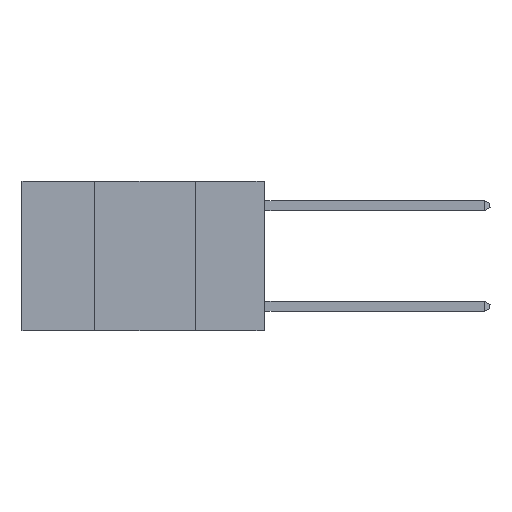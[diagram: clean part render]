
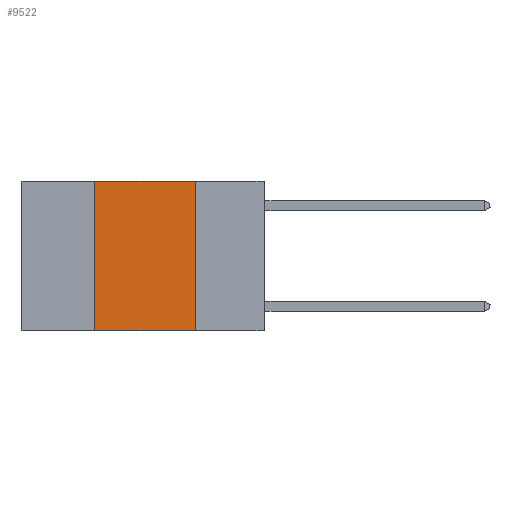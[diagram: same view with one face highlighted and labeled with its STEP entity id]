
A CAD part, left-side view. The second image highlights one B-rep face of the part: STEP entity #9522.
In plain terms, the highlighted planar face has unit normal (-1, 0, 0).
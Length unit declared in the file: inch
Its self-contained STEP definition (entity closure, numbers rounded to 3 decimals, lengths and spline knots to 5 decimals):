
#1008 = DIRECTION ( 'NONE',  ( 0., 0., 1. ) ) ;
#1187 = LINE ( 'NONE', #14145, #12394 ) ;
#1374 = ORIENTED_EDGE ( 'NONE', *, *, #8003, .F. ) ;
#2022 = EDGE_CURVE ( 'NONE', #8125, #4123, #12876, .T. ) ;
#2050 = LINE ( 'NONE', #7362, #14471 ) ;
#4123 = VERTEX_POINT ( 'NONE', #14188 ) ;
#4880 = DIRECTION ( 'NONE',  ( 1., 0., 0. ) ) ;
#5107 = AXIS2_PLACEMENT_3D ( 'NONE', #16831, #4880, #13001 ) ;
#5209 = DIRECTION ( 'NONE',  ( 0., -1., 0. ) ) ;
#7362 = CARTESIAN_POINT ( 'NONE',  ( 0., 0.17, 0. ) ) ;
#7756 = EDGE_CURVE ( 'NONE', #9076, #4123, #2050, .T. ) ;
#7764 = CARTESIAN_POINT ( 'NONE',  ( 0., 0.42, -0.37 ) ) ;
#8003 = EDGE_CURVE ( 'NONE', #8125, #15830, #10076, .T. ) ;
#8125 = VERTEX_POINT ( 'NONE', #7764 ) ;
#8781 = VECTOR ( 'NONE', #5209, 39.37008 ) ;
#9076 = VERTEX_POINT ( 'NONE', #15460 ) ;
#9171 = EDGE_CURVE ( 'NONE', #15830, #9076, #1187, .T. ) ;
#9522 = ADVANCED_FACE ( 'NONE', ( #11594 ), #16740, .F. ) ;
#9675 = VECTOR ( 'NONE', #1008, 39.37008 ) ;
#9993 = ORIENTED_EDGE ( 'NONE', *, *, #7756, .F. ) ;
#10076 = LINE ( 'NONE', #12842, #9675 ) ;
#10153 = CARTESIAN_POINT ( 'NONE',  ( 0., 0.42, 0. ) ) ;
#10262 = DIRECTION ( 'NONE',  ( 0., -1., 0. ) ) ;
#10273 = DIRECTION ( 'NONE',  ( 0., 0., -1. ) ) ;
#11594 = FACE_OUTER_BOUND ( 'NONE', #11990, .T. ) ;
#11990 = EDGE_LOOP ( 'NONE', ( #9993, #15850, #1374, #12882 ) ) ;
#12394 = VECTOR ( 'NONE', #10262, 39.37008 ) ;
#12842 = CARTESIAN_POINT ( 'NONE',  ( 0., 0.42, 0. ) ) ;
#12876 = LINE ( 'NONE', #14518, #8781 ) ;
#12882 = ORIENTED_EDGE ( 'NONE', *, *, #2022, .T. ) ;
#13001 = DIRECTION ( 'NONE',  ( 0., 0., -1. ) ) ;
#14145 = CARTESIAN_POINT ( 'NONE',  ( 0., 0.6, 0. ) ) ;
#14188 = CARTESIAN_POINT ( 'NONE',  ( 0., 0.17, -0.37 ) ) ;
#14471 = VECTOR ( 'NONE', #10273, 39.37008 ) ;
#14518 = CARTESIAN_POINT ( 'NONE',  ( 0., 0.6, -0.37 ) ) ;
#15460 = CARTESIAN_POINT ( 'NONE',  ( 0., 0.17, 0. ) ) ;
#15830 = VERTEX_POINT ( 'NONE', #10153 ) ;
#15850 = ORIENTED_EDGE ( 'NONE', *, *, #9171, .F. ) ;
#16740 = PLANE ( 'NONE',  #5107 ) ;
#16831 = CARTESIAN_POINT ( 'NONE',  ( 0., 0.6, 0. ) ) ;
